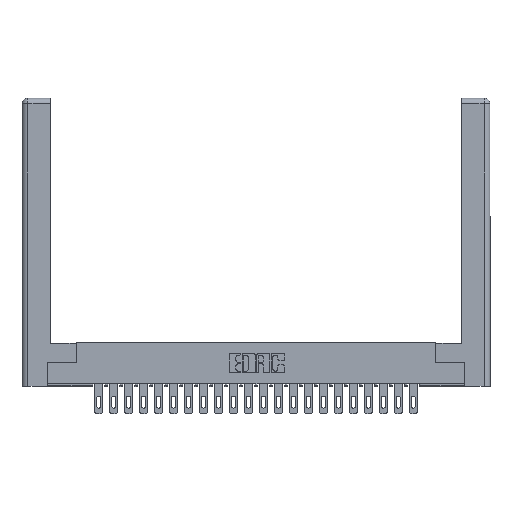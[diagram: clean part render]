
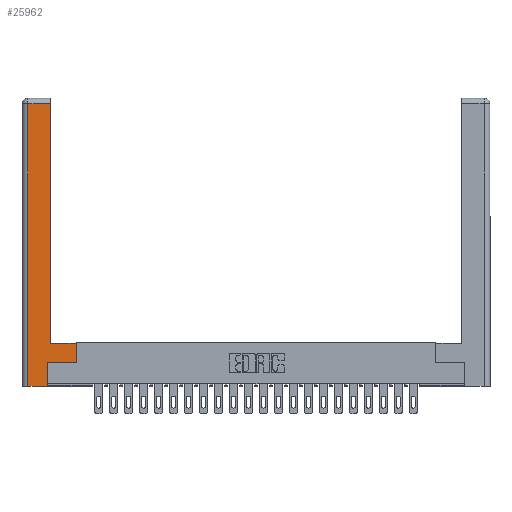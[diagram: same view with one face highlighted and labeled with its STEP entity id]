
A CAD part, top view. The second image highlights one B-rep face of the part: STEP entity #25962.
In plain terms, the highlighted planar face has unit normal (0, 0, 1).
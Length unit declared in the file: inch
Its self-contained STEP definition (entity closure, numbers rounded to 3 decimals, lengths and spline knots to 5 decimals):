
#3 = VECTOR ( 'NONE', #23830, 39.37008 ) ;
#67 = VERTEX_POINT ( 'NONE', #11005 ) ;
#739 = LINE ( 'NONE', #7677, #17861 ) ;
#747 = ORIENTED_EDGE ( 'NONE', *, *, #8384, .T. ) ;
#1166 = EDGE_CURVE ( 'NONE', #22908, #16655, #739, .T. ) ;
#2246 = DIRECTION ( 'NONE',  ( 0., 1., 0. ) ) ;
#2911 = CARTESIAN_POINT ( 'NONE',  ( 0.0615, 0., 0. ) ) ;
#3029 = DIRECTION ( 'NONE',  ( -1., 0., 0. ) ) ;
#3233 = EDGE_LOOP ( 'NONE', ( #23452, #16391, #11968, #4577, #747, #14575, #21733, #15071 ) ) ;
#3445 = CARTESIAN_POINT ( 'NONE',  ( 0.295, 2.94, 0. ) ) ;
#4290 = VECTOR ( 'NONE', #15323, 39.37008 ) ;
#4577 = ORIENTED_EDGE ( 'NONE', *, *, #17601, .T. ) ;
#6146 = CARTESIAN_POINT ( 'NONE',  ( 0.0615, 2.94, 0. ) ) ;
#6283 = CARTESIAN_POINT ( 'NONE',  ( 0.565, 0.245, 0. ) ) ;
#6944 = DIRECTION ( 'NONE',  ( 0., 1., 0. ) ) ;
#7228 = EDGE_CURVE ( 'NONE', #8808, #22908, #16444, .T. ) ;
#7248 = EDGE_CURVE ( 'NONE', #15454, #16676, #21981, .T. ) ;
#7488 = DIRECTION ( 'NONE',  ( -1., 0., 0. ) ) ;
#7677 = CARTESIAN_POINT ( 'NONE',  ( 0.295, 0.45, 0. ) ) ;
#8384 = EDGE_CURVE ( 'NONE', #25372, #26169, #17077, .T. ) ;
#8731 = CARTESIAN_POINT ( 'NONE',  ( 0.265, 0., 0. ) ) ;
#8808 = VERTEX_POINT ( 'NONE', #15191 ) ;
#10389 = LINE ( 'NONE', #6283, #14223 ) ;
#10469 = PLANE ( 'NONE',  #21552 ) ;
#10809 = FACE_OUTER_BOUND ( 'NONE', #3233, .T. ) ;
#10967 = LINE ( 'NONE', #8731, #4290 ) ;
#11005 = CARTESIAN_POINT ( 'NONE',  ( 0.0615, 0., 0. ) ) ;
#11716 = VECTOR ( 'NONE', #19072, 39.37008 ) ;
#11892 = CARTESIAN_POINT ( 'NONE',  ( 0.565, 0.45, 0. ) ) ;
#11968 = ORIENTED_EDGE ( 'NONE', *, *, #28482, .T. ) ;
#12132 = LINE ( 'NONE', #17947, #23193 ) ;
#14223 = VECTOR ( 'NONE', #21907, 39.37008 ) ;
#14575 = ORIENTED_EDGE ( 'NONE', *, *, #15683, .T. ) ;
#14855 = CARTESIAN_POINT ( 'NONE',  ( 0., 0., 0. ) ) ;
#15071 = ORIENTED_EDGE ( 'NONE', *, *, #1166, .T. ) ;
#15191 = CARTESIAN_POINT ( 'NONE',  ( 0.565, 0.245, 0. ) ) ;
#15323 = DIRECTION ( 'NONE',  ( 1., 0., 0. ) ) ;
#15427 = CARTESIAN_POINT ( 'NONE',  ( 0.265, 0.245, 0. ) ) ;
#15454 = VERTEX_POINT ( 'NONE', #3445 ) ;
#15683 = EDGE_CURVE ( 'NONE', #26169, #8808, #10389, .T. ) ;
#16391 = ORIENTED_EDGE ( 'NONE', *, *, #7248, .T. ) ;
#16444 = LINE ( 'NONE', #17340, #3 ) ;
#16634 = CARTESIAN_POINT ( 'NONE',  ( 0.265, 0., 0. ) ) ;
#16655 = VERTEX_POINT ( 'NONE', #27452 ) ;
#16676 = VERTEX_POINT ( 'NONE', #25204 ) ;
#17077 = LINE ( 'NONE', #28877, #22252 ) ;
#17340 = CARTESIAN_POINT ( 'NONE',  ( 0.565, 0.45, 0. ) ) ;
#17435 = DIRECTION ( 'NONE',  ( -1., 0., 0. ) ) ;
#17601 = EDGE_CURVE ( 'NONE', #67, #25372, #10967, .T. ) ;
#17861 = VECTOR ( 'NONE', #7488, 39.37008 ) ;
#17947 = CARTESIAN_POINT ( 'NONE',  ( 0.295, 3., 0. ) ) ;
#19072 = DIRECTION ( 'NONE',  ( 0., -1., 0. ) ) ;
#21552 = AXIS2_PLACEMENT_3D ( 'NONE', #14855, #25998, #3029 ) ;
#21733 = ORIENTED_EDGE ( 'NONE', *, *, #7228, .T. ) ;
#21907 = DIRECTION ( 'NONE',  ( 1., 0., 0. ) ) ;
#21981 = LINE ( 'NONE', #6146, #22311 ) ;
#22252 = VECTOR ( 'NONE', #2246, 39.37008 ) ;
#22311 = VECTOR ( 'NONE', #17435, 39.37008 ) ;
#22908 = VERTEX_POINT ( 'NONE', #11892 ) ;
#23110 = LINE ( 'NONE', #2911, #11716 ) ;
#23193 = VECTOR ( 'NONE', #6944, 39.37008 ) ;
#23452 = ORIENTED_EDGE ( 'NONE', *, *, #27599, .T. ) ;
#23830 = DIRECTION ( 'NONE',  ( 0., 1., 0. ) ) ;
#25204 = CARTESIAN_POINT ( 'NONE',  ( 0.0615, 2.94, 0. ) ) ;
#25372 = VERTEX_POINT ( 'NONE', #16634 ) ;
#25962 = ADVANCED_FACE ( 'NONE', ( #10809 ), #10469, .F. ) ;
#25998 = DIRECTION ( 'NONE',  ( 0., 0., -1. ) ) ;
#26169 = VERTEX_POINT ( 'NONE', #15427 ) ;
#27452 = CARTESIAN_POINT ( 'NONE',  ( 0.295, 0.45, 0. ) ) ;
#27599 = EDGE_CURVE ( 'NONE', #16655, #15454, #12132, .T. ) ;
#28482 = EDGE_CURVE ( 'NONE', #16676, #67, #23110, .T. ) ;
#28877 = CARTESIAN_POINT ( 'NONE',  ( 0.265, 0.245, 0. ) ) ;
